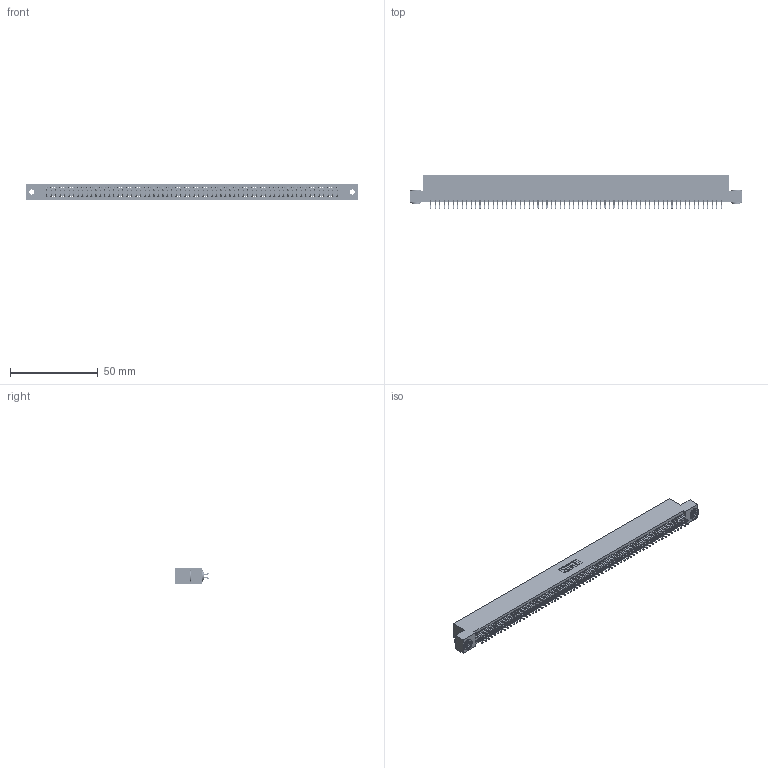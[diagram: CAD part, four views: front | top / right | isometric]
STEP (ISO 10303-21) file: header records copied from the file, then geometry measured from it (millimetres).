
FILE_DESCRIPTION (( 'STEP AP203' ), '1' );
FILE_NAME ('345-132-556-203.STEP', '2019-11-07T22:26:40', ( '' ), ( '' ), 'SwSTEP 2.0', 'SolidWorks 2016', '' );
FILE_SCHEMA (( 'CONFIG_CONTROL_DESIGN' ));
Length unit declared in the file: inch
Products named in the file (4): 345-132-556-203; 345-250-002_345-250-002-102; 345 Part_Flush Mounting Lugs - 0.156 Dia-TH; 345-292-001_556 Tail
Assembly tree (135 placements, depth 2):
  345-132-556-203
    345 Part_Flush Mounting Lugs - 0.156 Dia-TH
    345-292-001_556 Tail  x132
    345-250-002_345-250-002-102  x2
Bounding box: 188.85 x 19.24 x 9.4 mm (x, y, z)
Volume: 18581.9 mm3; surface area: 28021.4 mm2
Topology: 135 solids, 135 shells, 7556 faces, 22461 edges, 14794 vertices
Faces by surface type: plane 4974, cylinder 2574, cone 8
Entity records: 49424 total; most frequent: CARTESIAN_POINT 8251, ORIENTED_EDGE 8166, DIRECTION 7265, EDGE_CURVE 4083, LINE 3655, VECTOR 3655, VERTEX_POINT 2718, AXIS2_PLACEMENT_3D 1805
